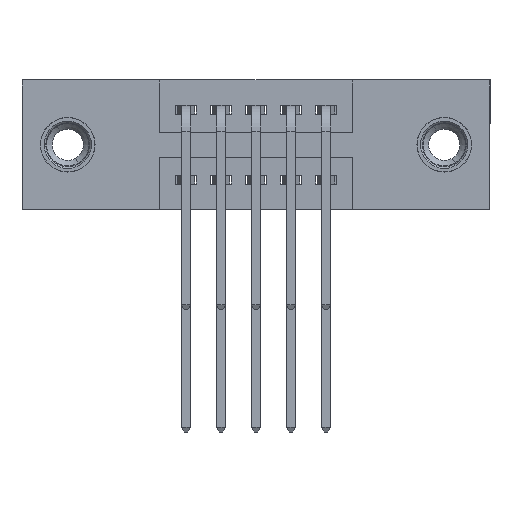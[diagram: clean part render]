
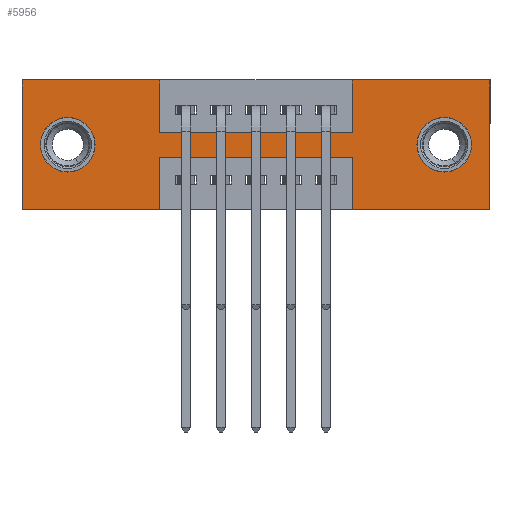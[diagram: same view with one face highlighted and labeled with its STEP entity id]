
A CAD part, front view. The second image highlights one B-rep face of the part: STEP entity #5956.
In plain terms, the highlighted planar face has unit normal (0, -1, 0).
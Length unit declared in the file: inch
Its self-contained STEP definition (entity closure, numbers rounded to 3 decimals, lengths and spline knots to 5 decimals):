
#81 = CARTESIAN_POINT ( 'NONE',  ( 1.335, 0., 0. ) ) ;
#110 = EDGE_LOOP ( 'NONE', ( #4961, #9772 ) ) ;
#437 = EDGE_LOOP ( 'NONE', ( #9356, #9152 ) ) ;
#473 = VERTEX_POINT ( 'NONE', #2653 ) ;
#477 = AXIS2_PLACEMENT_3D ( 'NONE', #12493, #669, #715 ) ;
#653 = CARTESIAN_POINT ( 'NONE',  ( 1.205, 0., -0.107 ) ) ;
#669 = DIRECTION ( 'NONE',  ( 0., 1., 0. ) ) ;
#678 = CARTESIAN_POINT ( 'NONE',  ( 0.9425, 0., 0. ) ) ;
#715 = DIRECTION ( 'NONE',  ( 0., 0., 1. ) ) ;
#940 = DIRECTION ( 'NONE',  ( 0., 0., 1. ) ) ;
#941 = CARTESIAN_POINT ( 'NONE',  ( 1.205, 0., -0.185 ) ) ;
#942 = CARTESIAN_POINT ( 'NONE',  ( 1.205, 0., -0.263 ) ) ;
#994 = DIRECTION ( 'NONE',  ( 0., 0., -1. ) ) ;
#1134 = EDGE_CURVE ( 'NONE', #12721, #5798, #11696, .T. ) ;
#1217 = AXIS2_PLACEMENT_3D ( 'NONE', #7753, #2833, #940 ) ;
#1336 = EDGE_CURVE ( 'NONE', #5798, #12319, #6032, .T. ) ;
#1501 = VERTEX_POINT ( 'NONE', #11564 ) ;
#1606 = LINE ( 'NONE', #2836, #6534 ) ;
#1671 = DIRECTION ( 'NONE',  ( 0., 0., 1. ) ) ;
#1757 = VERTEX_POINT ( 'NONE', #4424 ) ;
#1850 = LINE ( 'NONE', #5700, #9080 ) ;
#1986 = ORIENTED_EDGE ( 'NONE', *, *, #12649, .F. ) ;
#2110 = DIRECTION ( 'NONE',  ( 0., 0., -1. ) ) ;
#2230 = LINE ( 'NONE', #9936, #4671 ) ;
#2239 = CARTESIAN_POINT ( 'NONE',  ( 0.13, 0., -0.107 ) ) ;
#2607 = EDGE_CURVE ( 'NONE', #12574, #10591, #3906, .T. ) ;
#2626 = ORIENTED_EDGE ( 'NONE', *, *, #8389, .F. ) ;
#2653 = CARTESIAN_POINT ( 'NONE',  ( 1.335, 0., -0.37 ) ) ;
#2794 = CARTESIAN_POINT ( 'NONE',  ( 0.13, 0., -0.263 ) ) ;
#2833 = DIRECTION ( 'NONE',  ( 0., 1., 0. ) ) ;
#2836 = CARTESIAN_POINT ( 'NONE',  ( 0., 0., -0.37 ) ) ;
#2964 = EDGE_CURVE ( 'NONE', #12539, #9013, #10828, .T. ) ;
#2998 = ORIENTED_EDGE ( 'NONE', *, *, #8974, .F. ) ;
#3350 = LINE ( 'NONE', #4555, #7790 ) ;
#3439 = CARTESIAN_POINT ( 'NONE',  ( 0.3925, 0., -0.37 ) ) ;
#3523 = CIRCLE ( 'NONE', #477, 0.078 ) ;
#3642 = AXIS2_PLACEMENT_3D ( 'NONE', #941, #11975, #3809 ) ;
#3809 = DIRECTION ( 'NONE',  ( 0., 0., -1. ) ) ;
#3823 = DIRECTION ( 'NONE',  ( 0., 0., -1. ) ) ;
#3906 = CIRCLE ( 'NONE', #3642, 0.078 ) ;
#4182 = VERTEX_POINT ( 'NONE', #4481 ) ;
#4424 = CARTESIAN_POINT ( 'NONE',  ( 0.9425, 0., -0.15 ) ) ;
#4481 = CARTESIAN_POINT ( 'NONE',  ( 0., 0., -0.37 ) ) ;
#4547 = CARTESIAN_POINT ( 'NONE',  ( 0., 0., 0. ) ) ;
#4555 = CARTESIAN_POINT ( 'NONE',  ( 0.3925, 0., -0.15 ) ) ;
#4671 = VECTOR ( 'NONE', #2110, 39.37008 ) ;
#4961 = ORIENTED_EDGE ( 'NONE', *, *, #5095, .T. ) ;
#5061 = DIRECTION ( 'NONE',  ( 1., 0., 0. ) ) ;
#5095 = EDGE_CURVE ( 'NONE', #10591, #12574, #6313, .T. ) ;
#5213 = ORIENTED_EDGE ( 'NONE', *, *, #1336, .F. ) ;
#5383 = LINE ( 'NONE', #10519, #9553 ) ;
#5533 = DIRECTION ( 'NONE',  ( 0., 0., -1. ) ) ;
#5692 = EDGE_CURVE ( 'NONE', #473, #8391, #6757, .T. ) ;
#5700 = CARTESIAN_POINT ( 'NONE',  ( 0., 0., 0. ) ) ;
#5781 = VECTOR ( 'NONE', #12471, 39.37008 ) ;
#5798 = VERTEX_POINT ( 'NONE', #10608 ) ;
#5956 = ADVANCED_FACE ( 'NONE', ( #10621, #8602, #8108 ), #11242, .T. ) ;
#5985 = VERTEX_POINT ( 'NONE', #81 ) ;
#6032 = LINE ( 'NONE', #8772, #11417 ) ;
#6131 = ORIENTED_EDGE ( 'NONE', *, *, #11803, .F. ) ;
#6300 = DIRECTION ( 'NONE',  ( 0., -1., 0. ) ) ;
#6313 = CIRCLE ( 'NONE', #11046, 0.078 ) ;
#6448 = LINE ( 'NONE', #7914, #7656 ) ;
#6534 = VECTOR ( 'NONE', #7755, 39.37008 ) ;
#6709 = VECTOR ( 'NONE', #1671, 39.37008 ) ;
#6757 = LINE ( 'NONE', #10071, #7660 ) ;
#7218 = ORIENTED_EDGE ( 'NONE', *, *, #5692, .F. ) ;
#7487 = VERTEX_POINT ( 'NONE', #7609 ) ;
#7609 = CARTESIAN_POINT ( 'NONE',  ( 0.3925, 0., -0.22 ) ) ;
#7639 = DIRECTION ( 'NONE',  ( 0., 0., 1. ) ) ;
#7652 = CARTESIAN_POINT ( 'NONE',  ( 0.9425, 0., 0. ) ) ;
#7656 = VECTOR ( 'NONE', #11444, 39.37008 ) ;
#7660 = VECTOR ( 'NONE', #12258, 39.37008 ) ;
#7753 = CARTESIAN_POINT ( 'NONE',  ( 0.13, 0., -0.185 ) ) ;
#7755 = DIRECTION ( 'NONE',  ( -1., 0., 0. ) ) ;
#7790 = VECTOR ( 'NONE', #8364, 39.37008 ) ;
#7914 = CARTESIAN_POINT ( 'NONE',  ( 0.3925, 0., -0.37 ) ) ;
#7926 = EDGE_CURVE ( 'NONE', #5985, #473, #2230, .T. ) ;
#8058 = EDGE_CURVE ( 'NONE', #8148, #5985, #10710, .T. ) ;
#8108 = FACE_OUTER_BOUND ( 'NONE', #8201, .T. ) ;
#8148 = VERTEX_POINT ( 'NONE', #7652 ) ;
#8201 = EDGE_LOOP ( 'NONE', ( #8905, #2626, #12265, #7218, #11786, #9131, #6131, #10005, #5213, #10810, #2998, #1986 ) ) ;
#8364 = DIRECTION ( 'NONE',  ( 1., 0., 0. ) ) ;
#8389 = EDGE_CURVE ( 'NONE', #1501, #7487, #9415, .T. ) ;
#8391 = VERTEX_POINT ( 'NONE', #9989 ) ;
#8397 = LINE ( 'NONE', #678, #6709 ) ;
#8602 = FACE_BOUND ( 'NONE', #437, .T. ) ;
#8690 = DIRECTION ( 'NONE',  ( 0., 0., 1. ) ) ;
#8772 = CARTESIAN_POINT ( 'NONE',  ( 0.3925, 0., 0. ) ) ;
#8905 = ORIENTED_EDGE ( 'NONE', *, *, #10077, .F. ) ;
#8974 = EDGE_CURVE ( 'NONE', #4182, #12721, #1850, .T. ) ;
#9013 = VERTEX_POINT ( 'NONE', #2239 ) ;
#9051 = VERTEX_POINT ( 'NONE', #3439 ) ;
#9080 = VECTOR ( 'NONE', #7639, 39.37008 ) ;
#9131 = ORIENTED_EDGE ( 'NONE', *, *, #8058, .F. ) ;
#9152 = ORIENTED_EDGE ( 'NONE', *, *, #2964, .T. ) ;
#9196 = CARTESIAN_POINT ( 'NONE',  ( 0., 0., 0. ) ) ;
#9356 = ORIENTED_EDGE ( 'NONE', *, *, #9776, .T. ) ;
#9400 = CARTESIAN_POINT ( 'NONE',  ( 0., 0., -0.37 ) ) ;
#9415 = LINE ( 'NONE', #12687, #10946 ) ;
#9553 = VECTOR ( 'NONE', #8690, 39.37008 ) ;
#9563 = EDGE_CURVE ( 'NONE', #8391, #1501, #5383, .T. ) ;
#9739 = DIRECTION ( 'NONE',  ( -1., 0., 0. ) ) ;
#9772 = ORIENTED_EDGE ( 'NONE', *, *, #2607, .T. ) ;
#9776 = EDGE_CURVE ( 'NONE', #9013, #12539, #3523, .T. ) ;
#9936 = CARTESIAN_POINT ( 'NONE',  ( 1.335, 0., 0. ) ) ;
#9989 = CARTESIAN_POINT ( 'NONE',  ( 0.9425, 0., -0.37 ) ) ;
#10005 = ORIENTED_EDGE ( 'NONE', *, *, #10598, .F. ) ;
#10071 = CARTESIAN_POINT ( 'NONE',  ( 0., 0., -0.37 ) ) ;
#10077 = EDGE_CURVE ( 'NONE', #7487, #9051, #6448, .T. ) ;
#10519 = CARTESIAN_POINT ( 'NONE',  ( 0.9425, 0., -0.37 ) ) ;
#10591 = VERTEX_POINT ( 'NONE', #653 ) ;
#10598 = EDGE_CURVE ( 'NONE', #12319, #1757, #3350, .T. ) ;
#10608 = CARTESIAN_POINT ( 'NONE',  ( 0.3925, 0., 0. ) ) ;
#10621 = FACE_BOUND ( 'NONE', #110, .T. ) ;
#10710 = LINE ( 'NONE', #4547, #5781 ) ;
#10810 = ORIENTED_EDGE ( 'NONE', *, *, #1134, .F. ) ;
#10828 = CIRCLE ( 'NONE', #1217, 0.078 ) ;
#10946 = VECTOR ( 'NONE', #9739, 39.37008 ) ;
#10952 = VECTOR ( 'NONE', #5061, 39.37008 ) ;
#10982 = CARTESIAN_POINT ( 'NONE',  ( 0., 0., 0. ) ) ;
#11046 = AXIS2_PLACEMENT_3D ( 'NONE', #11431, #11392, #5533 ) ;
#11070 = CARTESIAN_POINT ( 'NONE',  ( 0.3925, 0., -0.15 ) ) ;
#11142 = AXIS2_PLACEMENT_3D ( 'NONE', #9400, #6300, #3823 ) ;
#11242 = PLANE ( 'NONE',  #11142 ) ;
#11392 = DIRECTION ( 'NONE',  ( 0., 1., 0. ) ) ;
#11417 = VECTOR ( 'NONE', #994, 39.37008 ) ;
#11431 = CARTESIAN_POINT ( 'NONE',  ( 1.205, 0., -0.185 ) ) ;
#11444 = DIRECTION ( 'NONE',  ( 0., 0., -1. ) ) ;
#11564 = CARTESIAN_POINT ( 'NONE',  ( 0.9425, 0., -0.22 ) ) ;
#11696 = LINE ( 'NONE', #10982, #10952 ) ;
#11786 = ORIENTED_EDGE ( 'NONE', *, *, #7926, .F. ) ;
#11803 = EDGE_CURVE ( 'NONE', #1757, #8148, #8397, .T. ) ;
#11975 = DIRECTION ( 'NONE',  ( 0., 1., 0. ) ) ;
#12258 = DIRECTION ( 'NONE',  ( -1., 0., 0. ) ) ;
#12265 = ORIENTED_EDGE ( 'NONE', *, *, #9563, .F. ) ;
#12319 = VERTEX_POINT ( 'NONE', #11070 ) ;
#12471 = DIRECTION ( 'NONE',  ( 1., 0., 0. ) ) ;
#12493 = CARTESIAN_POINT ( 'NONE',  ( 0.13, 0., -0.185 ) ) ;
#12539 = VERTEX_POINT ( 'NONE', #2794 ) ;
#12574 = VERTEX_POINT ( 'NONE', #942 ) ;
#12649 = EDGE_CURVE ( 'NONE', #9051, #4182, #1606, .T. ) ;
#12687 = CARTESIAN_POINT ( 'NONE',  ( 0.3925, 0., -0.22 ) ) ;
#12721 = VERTEX_POINT ( 'NONE', #9196 ) ;
